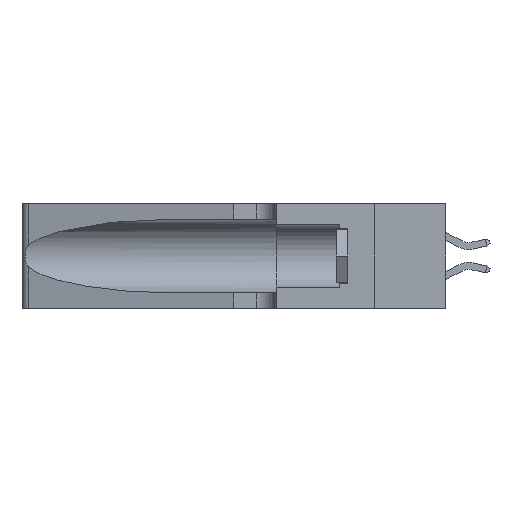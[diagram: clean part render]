
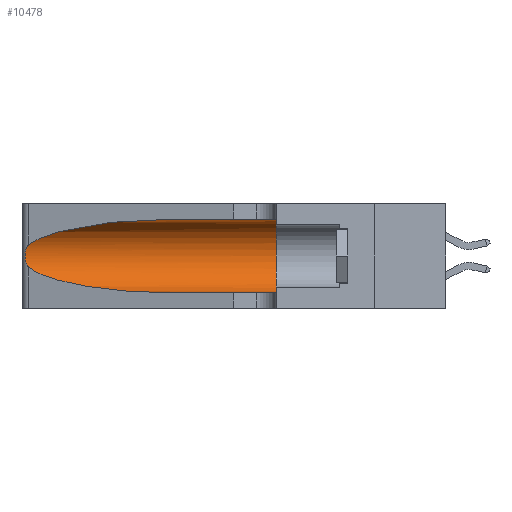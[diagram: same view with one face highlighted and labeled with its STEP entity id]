
A CAD part, left-side view. The second image highlights one B-rep face of the part: STEP entity #10478.
In plain terms, the highlighted cylindrical face has radius 3.308 mm (diameter 6.617 mm), a partial arc.
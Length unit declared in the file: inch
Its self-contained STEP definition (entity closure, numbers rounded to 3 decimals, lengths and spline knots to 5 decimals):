
#472 = CARTESIAN_POINT ( 'NONE',  ( 0.2373, 1.15595, 0.28018 ) ) ;
#637 =( BOUNDED_CURVE ( )  B_SPLINE_CURVE ( 3, ( #3269, #1727, #13838, #1583 ),
 .UNSPECIFIED., .F., .F. ) 
 B_SPLINE_CURVE_WITH_KNOTS ( ( 4, 4 ),
 ( 3.44316, 4.71239 ),
 .UNSPECIFIED. ) 
 CURVE ( )  GEOMETRIC_REPRESENTATION_ITEM ( )  RATIONAL_B_SPLINE_CURVE ( ( 1., 0.87, 0.87, 1. ) ) 
 REPRESENTATION_ITEM ( '' )  );
#1104 = EDGE_LOOP ( 'NONE', ( #13733, #3544, #18972, #2630, #10990, #3426 ) ) ;
#1139 = CARTESIAN_POINT ( 'NONE',  ( 0.25789, 1.23486, 0.15765 ) ) ;
#1583 = CARTESIAN_POINT ( 'NONE',  ( 0.1305, 0.72297, 0.05475 ) ) ;
#1727 = CARTESIAN_POINT ( 'NONE',  ( 0.2373, 1.15595, 0.08982 ) ) ;
#2148 = CARTESIAN_POINT ( 'NONE',  ( 0.1305, 0.72297, 0.31525 ) ) ;
#2289 = VERTEX_POINT ( 'NONE', #4928 ) ;
#2304 = B_SPLINE_CURVE_WITH_KNOTS ( 'NONE', 3,
 ( #8157, #11693, #15056, #21842, #11612, #11469, #10060, #18672, #8080, #2904, #1139, #20184, #21919, #11544 ),
 .UNSPECIFIED., .F., .F.,
 ( 4, 2, 2, 2, 2, 2, 4 ),
 ( 0., 0.00027, 0.00053, 0.00107, 0.0016, 0.00187, 0.00214 ),
 .UNSPECIFIED. ) ;
#2630 = ORIENTED_EDGE ( 'NONE', *, *, #20509, .T. ) ;
#2649 = CARTESIAN_POINT ( 'NONE',  ( 0.1305, 0.72297, 0.05475 ) ) ;
#2904 = CARTESIAN_POINT ( 'NONE',  ( 0.25856, 1.23593, 0.16098 ) ) ;
#2985 = DIRECTION ( 'NONE',  ( 0., -1., 0. ) ) ;
#3269 = CARTESIAN_POINT ( 'NONE',  ( 0.25487, 1.22718, 0.14631 ) ) ;
#3302 = VERTEX_POINT ( 'NONE', #2649 ) ;
#3426 = ORIENTED_EDGE ( 'NONE', *, *, #5202, .F. ) ;
#3544 = ORIENTED_EDGE ( 'NONE', *, *, #5932, .T. ) ;
#3829 = CARTESIAN_POINT ( 'NONE',  ( 0.25487, 1.22718, 0.22369 ) ) ;
#3924 = LINE ( 'NONE', #17073, #17186 ) ;
#4208 = CARTESIAN_POINT ( 'NONE',  ( 0.25487, 1.22718, 0.14631 ) ) ;
#4928 = CARTESIAN_POINT ( 'NONE',  ( 0.25487, 1.22718, 0.22369 ) ) ;
#5202 = EDGE_CURVE ( 'NONE', #11689, #12560, #3924, .T. ) ;
#5696 = CIRCLE ( 'NONE', #9199, 0.13025 ) ;
#5770 = CARTESIAN_POINT ( 'NONE',  ( 0.18966, 0.96281, 0.31525 ) ) ;
#5830 = AXIS2_PLACEMENT_3D ( 'NONE', #15119, #6335, #11599 ) ;
#5932 = EDGE_CURVE ( 'NONE', #2289, #9364, #2304, .T. ) ;
#6335 = DIRECTION ( 'NONE',  ( 0., -1., 0. ) ) ;
#8080 = CARTESIAN_POINT ( 'NONE',  ( 0.26017, 1.23833, 0.17102 ) ) ;
#8157 = CARTESIAN_POINT ( 'NONE',  ( 0.25487, 1.22718, 0.22369 ) ) ;
#8727 = CYLINDRICAL_SURFACE ( 'NONE', #5830, 0.13025 ) ;
#9199 = AXIS2_PLACEMENT_3D ( 'NONE', #21568, #14634, #21250 ) ;
#9364 = VERTEX_POINT ( 'NONE', #4208 ) ;
#10060 = CARTESIAN_POINT ( 'NONE',  ( 0.26075, 1.23896, 0.19203 ) ) ;
#10478 = ADVANCED_FACE ( 'NONE', ( #20384 ), #8727, .F. ) ;
#10990 = ORIENTED_EDGE ( 'NONE', *, *, #13834, .F. ) ;
#11117 = CARTESIAN_POINT ( 'NONE',  ( 0.1305, 0.72297, 0.31525 ) ) ;
#11469 = CARTESIAN_POINT ( 'NONE',  ( 0.26018, 1.23835, 0.19895 ) ) ;
#11544 = CARTESIAN_POINT ( 'NONE',  ( 0.25487, 1.22718, 0.14631 ) ) ;
#11599 = DIRECTION ( 'NONE',  ( 0., 0., -1. ) ) ;
#11612 = CARTESIAN_POINT ( 'NONE',  ( 0.25854, 1.2359, 0.20912 ) ) ;
#11689 = VERTEX_POINT ( 'NONE', #11117 ) ;
#11693 = CARTESIAN_POINT ( 'NONE',  ( 0.25555, 1.22994, 0.2215 ) ) ;
#12560 = VERTEX_POINT ( 'NONE', #20906 ) ;
#12653 = CARTESIAN_POINT ( 'NONE',  ( 0.1305, 0.35, 0.05475 ) ) ;
#13101 = VERTEX_POINT ( 'NONE', #12653 ) ;
#13148 = CARTESIAN_POINT ( 'NONE',  ( 0.1305, 1.61858, 0.05475 ) ) ;
#13681 = LINE ( 'NONE', #13148, #16360 ) ;
#13733 = ORIENTED_EDGE ( 'NONE', *, *, #19535, .T. ) ;
#13834 = EDGE_CURVE ( 'NONE', #12560, #13101, #5696, .T. ) ;
#13838 = CARTESIAN_POINT ( 'NONE',  ( 0.18966, 0.96281, 0.05475 ) ) ;
#14634 = DIRECTION ( 'NONE',  ( 0., 1., 0. ) ) ;
#15056 = CARTESIAN_POINT ( 'NONE',  ( 0.25639, 1.23184, 0.21858 ) ) ;
#15119 = CARTESIAN_POINT ( 'NONE',  ( 0.1305, 1.61858, 0.185 ) ) ;
#15195 = DIRECTION ( 'NONE',  ( 0., -1., 0. ) ) ;
#16360 = VECTOR ( 'NONE', #2985, 39.37008 ) ;
#16736 =( BOUNDED_CURVE ( )  B_SPLINE_CURVE ( 3, ( #2148, #5770, #472, #3829 ),
 .UNSPECIFIED., .F., .F. ) 
 B_SPLINE_CURVE_WITH_KNOTS ( ( 4, 4 ),
 ( 1.5708, 2.84003 ),
 .UNSPECIFIED. ) 
 CURVE ( )  GEOMETRIC_REPRESENTATION_ITEM ( )  RATIONAL_B_SPLINE_CURVE ( ( 1., 0.87, 0.87, 1. ) ) 
 REPRESENTATION_ITEM ( '' )  );
#17073 = CARTESIAN_POINT ( 'NONE',  ( 0.1305, 1.61858, 0.31525 ) ) ;
#17186 = VECTOR ( 'NONE', #15195, 39.37008 ) ;
#18672 = CARTESIAN_POINT ( 'NONE',  ( 0.26075, 1.23896, 0.178 ) ) ;
#18972 = ORIENTED_EDGE ( 'NONE', *, *, #21271, .T. ) ;
#19535 = EDGE_CURVE ( 'NONE', #11689, #2289, #16736, .T. ) ;
#20184 = CARTESIAN_POINT ( 'NONE',  ( 0.25639, 1.23186, 0.15144 ) ) ;
#20384 = FACE_OUTER_BOUND ( 'NONE', #1104, .T. ) ;
#20509 = EDGE_CURVE ( 'NONE', #3302, #13101, #13681, .T. ) ;
#20906 = CARTESIAN_POINT ( 'NONE',  ( 0.1305, 0.35, 0.31525 ) ) ;
#21250 = DIRECTION ( 'NONE',  ( 0., 0., 1. ) ) ;
#21271 = EDGE_CURVE ( 'NONE', #9364, #3302, #637, .T. ) ;
#21568 = CARTESIAN_POINT ( 'NONE',  ( 0.1305, 0.35, 0.185 ) ) ;
#21842 = CARTESIAN_POINT ( 'NONE',  ( 0.25787, 1.23484, 0.2124 ) ) ;
#21919 = CARTESIAN_POINT ( 'NONE',  ( 0.25555, 1.22993, 0.14849 ) ) ;
